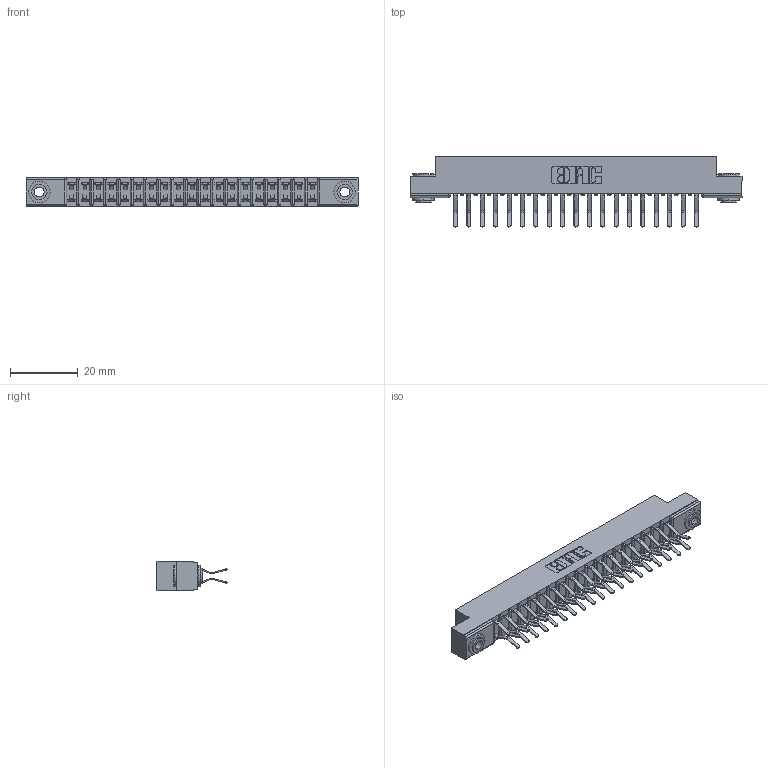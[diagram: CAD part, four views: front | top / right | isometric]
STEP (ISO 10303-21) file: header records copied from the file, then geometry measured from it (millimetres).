
FILE_DESCRIPTION (( 'STEP AP203' ), '1' );
FILE_NAME ('357-038-460-203.STEP', '2020-10-03T20:00:20', ( '' ), ( '' ), 'SwSTEP 2.0', 'SolidWorks 2020', '' );
FILE_SCHEMA (( 'CONFIG_CONTROL_DESIGN' ));
Length unit declared in the file: inch
Products named in the file (4): 345-250-002_345-250-002-102; 307 Part_.156 Dia Mounting Holes; 307-290-001_560; 357-038-460-203
Assembly tree (41 placements, depth 2):
  357-038-460-203
    307 Part_.156 Dia Mounting Holes
    307-290-001_560  x38
    345-250-002_345-250-002-102  x2
Bounding box: 98.3 x 20.73 x 8.71 mm (x, y, z)
Volume: 6478.7 mm3; surface area: 11821.5 mm2
Topology: 41 solids, 41 shells, 2090 faces, 5831 edges, 3778 vertices
Faces by surface type: plane 1348, cylinder 694, sphere 40, cone 8
Entity records: 20901 total; most frequent: CARTESIAN_POINT 3408, ORIENTED_EDGE 3366, DIRECTION 3363, EDGE_CURVE 1683, VECTOR 1273, LINE 1273, VERTEX_POINT 1090, AXIS2_PLACEMENT_3D 1045
